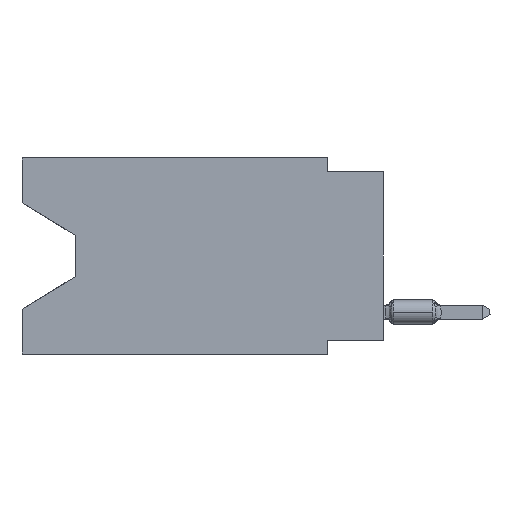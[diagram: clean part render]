
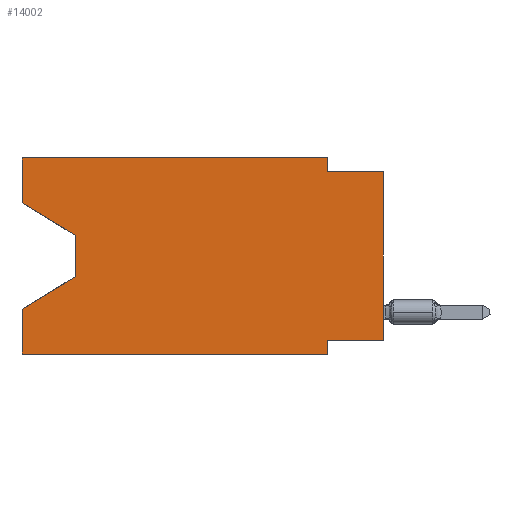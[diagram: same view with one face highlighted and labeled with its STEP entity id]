
A CAD part, left-side view. The second image highlights one B-rep face of the part: STEP entity #14002.
In plain terms, the highlighted planar face has unit normal (-1, 0, 0).
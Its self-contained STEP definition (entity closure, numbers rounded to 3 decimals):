
#741 = CARTESIAN_POINT ( 'NONE',  ( 0., 16.383, -8.89 ) ) ;
#1180 = VERTEX_POINT ( 'NONE', #51684 ) ;
#2453 = EDGE_CURVE ( 'NONE', #4840, #4340, #58245, .T. ) ;
#3109 = ORIENTED_EDGE ( 'NONE', *, *, #62979, .T. ) ;
#3471 = LINE ( 'NONE', #14596, #50558 ) ;
#4067 = EDGE_CURVE ( 'NONE', #63082, #33880, #44972, .T. ) ;
#4183 = DIRECTION ( 'NONE',  ( 0., -1., 0. ) ) ;
#4340 = VERTEX_POINT ( 'NONE', #30873 ) ;
#4491 = CARTESIAN_POINT ( 'NONE',  ( 0., 0., -0.635 ) ) ;
#4840 = VERTEX_POINT ( 'NONE', #42245 ) ;
#5625 = CARTESIAN_POINT ( 'NONE',  ( 0., 16.383, 0. ) ) ;
#6148 = DIRECTION ( 'NONE',  ( 0., -0.855, -0.519 ) ) ;
#6984 = VECTOR ( 'NONE', #39745, 1000. ) ;
#7130 = CARTESIAN_POINT ( 'NONE',  ( 0., 16.383, -2.038 ) ) ;
#7871 = ORIENTED_EDGE ( 'NONE', *, *, #63078, .F. ) ;
#9895 = LINE ( 'NONE', #5625, #29830 ) ;
#10284 = DIRECTION ( 'NONE',  ( 0., 1., 0. ) ) ;
#10446 = CARTESIAN_POINT ( 'NONE',  ( 0., 0., 0. ) ) ;
#10840 = DIRECTION ( 'NONE',  ( 0., 0., -1. ) ) ;
#11829 = CARTESIAN_POINT ( 'NONE',  ( 0., 13.97, -3.505 ) ) ;
#12024 = LINE ( 'NONE', #7130, #15567 ) ;
#12518 = ORIENTED_EDGE ( 'NONE', *, *, #20946, .T. ) ;
#14002 = ADVANCED_FACE ( 'NONE', ( #48264 ), #23359, .F. ) ;
#14466 = EDGE_CURVE ( 'NONE', #63034, #43659, #9895, .T. ) ;
#14596 = CARTESIAN_POINT ( 'NONE',  ( 0., 2.54, -8.89 ) ) ;
#14839 = CARTESIAN_POINT ( 'NONE',  ( 0., 2.54, 0. ) ) ;
#15567 = VECTOR ( 'NONE', #6148, 1000. ) ;
#17530 = EDGE_CURVE ( 'NONE', #43659, #63082, #19898, .T. ) ;
#17750 = VERTEX_POINT ( 'NONE', #4491 ) ;
#17916 = ORIENTED_EDGE ( 'NONE', *, *, #4067, .F. ) ;
#18441 = CARTESIAN_POINT ( 'NONE',  ( 0., 16.383, 0. ) ) ;
#19898 = LINE ( 'NONE', #44485, #50009 ) ;
#20424 = VECTOR ( 'NONE', #58878, 1000. ) ;
#20751 = LINE ( 'NONE', #26351, #35283 ) ;
#20946 = EDGE_CURVE ( 'NONE', #31637, #41804, #20999, .T. ) ;
#20999 = LINE ( 'NONE', #11829, #35244 ) ;
#21376 = DIRECTION ( 'NONE',  ( 0., -1., 0. ) ) ;
#22073 = ORIENTED_EDGE ( 'NONE', *, *, #17530, .F. ) ;
#22480 = EDGE_CURVE ( 'NONE', #57679, #1180, #20751, .T. ) ;
#22839 = CARTESIAN_POINT ( 'NONE',  ( 0., 2.54, 0. ) ) ;
#23359 = PLANE ( 'NONE',  #25017 ) ;
#24101 = DIRECTION ( 'NONE',  ( 0., 0., -1. ) ) ;
#24565 = DIRECTION ( 'NONE',  ( 0., 0., 1. ) ) ;
#25017 = AXIS2_PLACEMENT_3D ( 'NONE', #18441, #37482, #58749 ) ;
#25453 = ORIENTED_EDGE ( 'NONE', *, *, #14466, .F. ) ;
#25684 = ORIENTED_EDGE ( 'NONE', *, *, #51345, .T. ) ;
#26351 = CARTESIAN_POINT ( 'NONE',  ( 0., 0., -8.255 ) ) ;
#27645 = VECTOR ( 'NONE', #24565, 1000. ) ;
#29830 = VECTOR ( 'NONE', #30230, 1000. ) ;
#29933 = ORIENTED_EDGE ( 'NONE', *, *, #63729, .T. ) ;
#30230 = DIRECTION ( 'NONE',  ( 0., 0., 1. ) ) ;
#30873 = CARTESIAN_POINT ( 'NONE',  ( 0., 16.383, -6.852 ) ) ;
#31637 = VERTEX_POINT ( 'NONE', #36139 ) ;
#31847 = VECTOR ( 'NONE', #61176, 1000. ) ;
#32547 = ORIENTED_EDGE ( 'NONE', *, *, #50830, .T. ) ;
#33393 = CARTESIAN_POINT ( 'NONE',  ( 0., 2.54, -0.635 ) ) ;
#33880 = VERTEX_POINT ( 'NONE', #33393 ) ;
#35244 = VECTOR ( 'NONE', #10840, 1000. ) ;
#35283 = VECTOR ( 'NONE', #10284, 1000. ) ;
#35992 = LINE ( 'NONE', #10446, #27645 ) ;
#36139 = CARTESIAN_POINT ( 'NONE',  ( 0., 13.97, -3.505 ) ) ;
#37482 = DIRECTION ( 'NONE',  ( 1., 0., 0. ) ) ;
#38240 = ORIENTED_EDGE ( 'NONE', *, *, #2453, .F. ) ;
#38843 = EDGE_CURVE ( 'NONE', #1180, #41626, #3471, .T. ) ;
#39615 = VECTOR ( 'NONE', #58232, 1000. ) ;
#39712 = VECTOR ( 'NONE', #21376, 1000. ) ;
#39745 = DIRECTION ( 'NONE',  ( 0., 0., -1. ) ) ;
#40718 = LINE ( 'NONE', #741, #39712 ) ;
#41626 = VERTEX_POINT ( 'NONE', #59634 ) ;
#41804 = VERTEX_POINT ( 'NONE', #57624 ) ;
#42245 = CARTESIAN_POINT ( 'NONE',  ( 0., 16.383, -8.89 ) ) ;
#43659 = VERTEX_POINT ( 'NONE', #44734 ) ;
#44485 = CARTESIAN_POINT ( 'NONE',  ( 0., 16.383, 0. ) ) ;
#44734 = CARTESIAN_POINT ( 'NONE',  ( 0., 16.383, 0. ) ) ;
#44972 = LINE ( 'NONE', #14839, #6984 ) ;
#48264 = FACE_OUTER_BOUND ( 'NONE', #51982, .T. ) ;
#50009 = VECTOR ( 'NONE', #4183, 1000. ) ;
#50558 = VECTOR ( 'NONE', #24101, 1000. ) ;
#50830 = EDGE_CURVE ( 'NONE', #57679, #17750, #35992, .T. ) ;
#51008 = LINE ( 'NONE', #52309, #31847 ) ;
#51345 = EDGE_CURVE ( 'NONE', #41804, #4340, #51008, .T. ) ;
#51684 = CARTESIAN_POINT ( 'NONE',  ( 0., 2.54, -8.255 ) ) ;
#51982 = EDGE_LOOP ( 'NONE', ( #3109, #12518, #25684, #38240, #29933, #58021, #54511, #32547, #7871, #17916, #22073, #25453 ) ) ;
#52309 = CARTESIAN_POINT ( 'NONE',  ( 0., 13.97, -5.385 ) ) ;
#52997 = CARTESIAN_POINT ( 'NONE',  ( 0., 16.383, 0. ) ) ;
#53300 = LINE ( 'NONE', #57903, #39615 ) ;
#54511 = ORIENTED_EDGE ( 'NONE', *, *, #22480, .F. ) ;
#57624 = CARTESIAN_POINT ( 'NONE',  ( 0., 13.97, -5.385 ) ) ;
#57679 = VERTEX_POINT ( 'NONE', #59717 ) ;
#57903 = CARTESIAN_POINT ( 'NONE',  ( 0., 0., -0.635 ) ) ;
#58021 = ORIENTED_EDGE ( 'NONE', *, *, #38843, .F. ) ;
#58232 = DIRECTION ( 'NONE',  ( 0., -1., 0. ) ) ;
#58245 = LINE ( 'NONE', #52997, #20424 ) ;
#58550 = CARTESIAN_POINT ( 'NONE',  ( 0., 16.383, -2.038 ) ) ;
#58749 = DIRECTION ( 'NONE',  ( 0., 0., -1. ) ) ;
#58878 = DIRECTION ( 'NONE',  ( 0., 0., 1. ) ) ;
#59634 = CARTESIAN_POINT ( 'NONE',  ( 0., 2.54, -8.89 ) ) ;
#59717 = CARTESIAN_POINT ( 'NONE',  ( 0., 0., -8.255 ) ) ;
#61176 = DIRECTION ( 'NONE',  ( 0., 0.855, -0.519 ) ) ;
#62979 = EDGE_CURVE ( 'NONE', #63034, #31637, #12024, .T. ) ;
#63034 = VERTEX_POINT ( 'NONE', #58550 ) ;
#63078 = EDGE_CURVE ( 'NONE', #33880, #17750, #53300, .T. ) ;
#63082 = VERTEX_POINT ( 'NONE', #22839 ) ;
#63729 = EDGE_CURVE ( 'NONE', #4840, #41626, #40718, .T. ) ;
